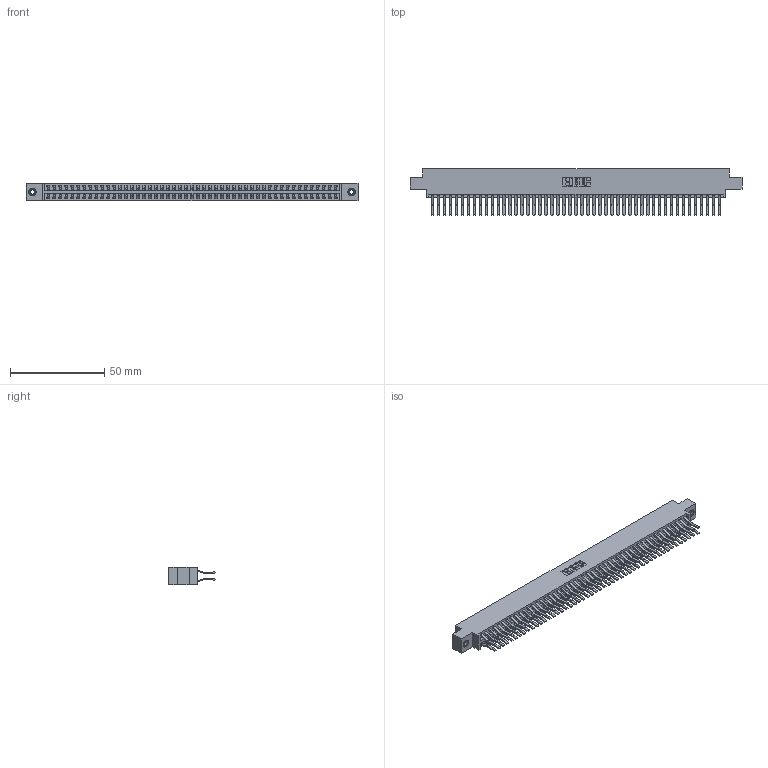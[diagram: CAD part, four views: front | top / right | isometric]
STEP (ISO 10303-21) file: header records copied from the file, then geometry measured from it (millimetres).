
FILE_DESCRIPTION (( 'STEP AP203' ), '1' );
FILE_NAME ('396-098-560-808.STEP', '2019-11-02T17:17:51', ( '' ), ( '' ), 'SwSTEP 2.0', 'SolidWorks 2016', '' );
FILE_SCHEMA (( 'CONFIG_CONTROL_DESIGN' ));
Length unit declared in the file: inch
Products named in the file (4): 396-098-560-808; 346 Part_0.170 Offset - 0.156 Dia-TI; 345-292-001_560 Tail; 345-250-001_345-250-003-102
Assembly tree (101 placements, depth 2):
  396-098-560-808
    346 Part_0.170 Offset - 0.156 Dia-TI
    345-292-001_560 Tail  x98
    345-250-001_345-250-003-102  x2
Bounding box: 176.15 x 24.78 x 9.4 mm (x, y, z)
Volume: 17712.3 mm3; surface area: 26370.2 mm2
Topology: 101 solids, 101 shells, 5478 faces, 16255 edges, 10698 vertices
Faces by surface type: plane 3542, cylinder 1920, cone 12, torus 4
Entity records: 32442 total; most frequent: CARTESIAN_POINT 5323, ORIENTED_EDGE 5250, DIRECTION 4771, EDGE_CURVE 2625, VECTOR 2273, LINE 2273, VERTEX_POINT 1744, AXIS2_PLACEMENT_3D 1249
